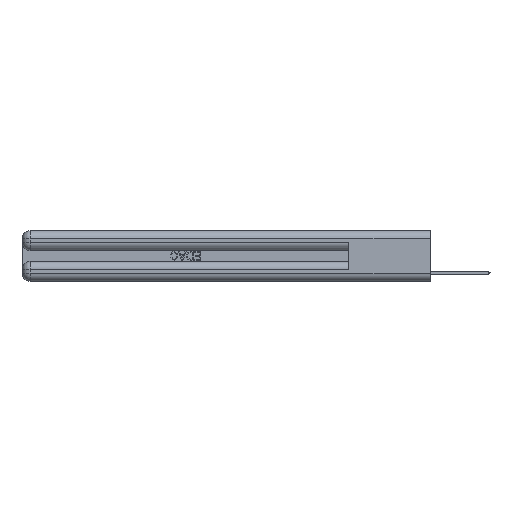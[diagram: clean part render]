
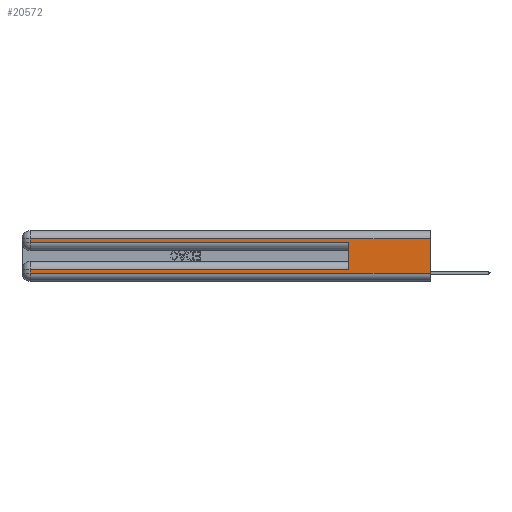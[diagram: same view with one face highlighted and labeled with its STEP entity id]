
A CAD part, left-side view. The second image highlights one B-rep face of the part: STEP entity #20572.
In plain terms, the highlighted planar face has unit normal (-1, 0, 0).
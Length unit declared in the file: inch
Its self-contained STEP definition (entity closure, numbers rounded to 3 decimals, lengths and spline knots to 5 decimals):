
#384 = VERTEX_POINT ( 'NONE', #10574 ) ;
#1027 = AXIS2_PLACEMENT_3D ( 'NONE', #28864, #4680, #23284 ) ;
#1366 = ORIENTED_EDGE ( 'NONE', *, *, #20256, .T. ) ;
#1648 = EDGE_CURVE ( 'NONE', #28261, #14164, #5357, .T. ) ;
#1990 = DIRECTION ( 'NONE',  ( 0., 0., -1. ) ) ;
#2284 = DIRECTION ( 'NONE',  ( 0., 0., -1. ) ) ;
#2775 = ORIENTED_EDGE ( 'NONE', *, *, #5877, .T. ) ;
#3923 = EDGE_CURVE ( 'NONE', #12205, #14164, #28699, .T. ) ;
#3982 = CARTESIAN_POINT ( 'NONE',  ( 0., 2.94, 0.31 ) ) ;
#4660 = VERTEX_POINT ( 'NONE', #22169 ) ;
#4680 = DIRECTION ( 'NONE',  ( 1., 0., 0. ) ) ;
#4927 = DIRECTION ( 'NONE',  ( 0., -1., 0. ) ) ;
#5206 = DIRECTION ( 'NONE',  ( 0., -1., 0. ) ) ;
#5357 = LINE ( 'NONE', #21335, #30252 ) ;
#5493 = VECTOR ( 'NONE', #1990, 39.37008 ) ;
#5877 = EDGE_CURVE ( 'NONE', #4660, #12205, #28928, .T. ) ;
#6397 = CARTESIAN_POINT ( 'NONE',  ( 0., 2.94, 0.06 ) ) ;
#6908 = CARTESIAN_POINT ( 'NONE',  ( 0., 0.6, 0.145 ) ) ;
#7137 = EDGE_CURVE ( 'NONE', #17621, #7567, #26832, .T. ) ;
#7164 = DIRECTION ( 'NONE',  ( 0., 1., 0. ) ) ;
#7239 = DIRECTION ( 'NONE',  ( 0., 1., 0. ) ) ;
#7567 = VERTEX_POINT ( 'NONE', #26624 ) ;
#7925 = LINE ( 'NONE', #21285, #10143 ) ;
#9041 = ORIENTED_EDGE ( 'NONE', *, *, #27137, .T. ) ;
#9960 = CARTESIAN_POINT ( 'NONE',  ( 0., 0., 0.31 ) ) ;
#10143 = VECTOR ( 'NONE', #7239, 39.37008 ) ;
#10389 = DIRECTION ( 'NONE',  ( 0., 0., 1. ) ) ;
#10574 = CARTESIAN_POINT ( 'NONE',  ( 0., 0.6, 0.085 ) ) ;
#10861 = CARTESIAN_POINT ( 'NONE',  ( 0., 0., 0.285 ) ) ;
#11038 = EDGE_LOOP ( 'NONE', ( #28624, #1366, #9041, #33844, #33009, #12537, #2775, #17057 ) ) ;
#11100 = VECTOR ( 'NONE', #7164, 39.37008 ) ;
#12034 = CARTESIAN_POINT ( 'NONE',  ( 0., 0., 0.31 ) ) ;
#12205 = VERTEX_POINT ( 'NONE', #6397 ) ;
#12537 = ORIENTED_EDGE ( 'NONE', *, *, #25966, .T. ) ;
#13376 = LINE ( 'NONE', #32115, #5493 ) ;
#14164 = VERTEX_POINT ( 'NONE', #34275 ) ;
#16805 = FACE_OUTER_BOUND ( 'NONE', #11038, .T. ) ;
#17057 = ORIENTED_EDGE ( 'NONE', *, *, #3923, .T. ) ;
#17621 = VERTEX_POINT ( 'NONE', #29559 ) ;
#20094 = VECTOR ( 'NONE', #5206, 39.37008 ) ;
#20256 = EDGE_CURVE ( 'NONE', #28261, #20524, #25603, .T. ) ;
#20524 = VERTEX_POINT ( 'NONE', #3982 ) ;
#20572 = ADVANCED_FACE ( 'NONE', ( #16805 ), #27478, .F. ) ;
#21285 = CARTESIAN_POINT ( 'NONE',  ( 0., 0., 0.085 ) ) ;
#21335 = CARTESIAN_POINT ( 'NONE',  ( 0., 0., 0.37 ) ) ;
#22169 = CARTESIAN_POINT ( 'NONE',  ( 0., 2.94, 0.085 ) ) ;
#23284 = DIRECTION ( 'NONE',  ( 0., 0., -1. ) ) ;
#23696 = EDGE_CURVE ( 'NONE', #384, #7567, #30917, .T. ) ;
#24046 = CARTESIAN_POINT ( 'NONE',  ( 0., 2.94, 0.37 ) ) ;
#25603 = LINE ( 'NONE', #9960, #11100 ) ;
#25966 = EDGE_CURVE ( 'NONE', #384, #4660, #7925, .T. ) ;
#26624 = CARTESIAN_POINT ( 'NONE',  ( 0., 0.6, 0.285 ) ) ;
#26832 = LINE ( 'NONE', #10861, #27951 ) ;
#27137 = EDGE_CURVE ( 'NONE', #20524, #17621, #13376, .T. ) ;
#27478 = PLANE ( 'NONE',  #1027 ) ;
#27730 = DIRECTION ( 'NONE',  ( 0., 0., -1. ) ) ;
#27951 = VECTOR ( 'NONE', #4927, 39.37008 ) ;
#28261 = VERTEX_POINT ( 'NONE', #12034 ) ;
#28624 = ORIENTED_EDGE ( 'NONE', *, *, #1648, .F. ) ;
#28699 = LINE ( 'NONE', #29037, #20094 ) ;
#28864 = CARTESIAN_POINT ( 'NONE',  ( 0., 0., 0.37 ) ) ;
#28928 = LINE ( 'NONE', #24046, #32785 ) ;
#29037 = CARTESIAN_POINT ( 'NONE',  ( 0., 0., 0.06 ) ) ;
#29559 = CARTESIAN_POINT ( 'NONE',  ( 0., 2.94, 0.285 ) ) ;
#30252 = VECTOR ( 'NONE', #27730, 39.37008 ) ;
#30917 = LINE ( 'NONE', #6908, #32516 ) ;
#32115 = CARTESIAN_POINT ( 'NONE',  ( 0., 2.94, 0.37 ) ) ;
#32516 = VECTOR ( 'NONE', #10389, 39.37008 ) ;
#32785 = VECTOR ( 'NONE', #2284, 39.37008 ) ;
#33009 = ORIENTED_EDGE ( 'NONE', *, *, #23696, .F. ) ;
#33844 = ORIENTED_EDGE ( 'NONE', *, *, #7137, .T. ) ;
#34275 = CARTESIAN_POINT ( 'NONE',  ( 0., 0., 0.06 ) ) ;
